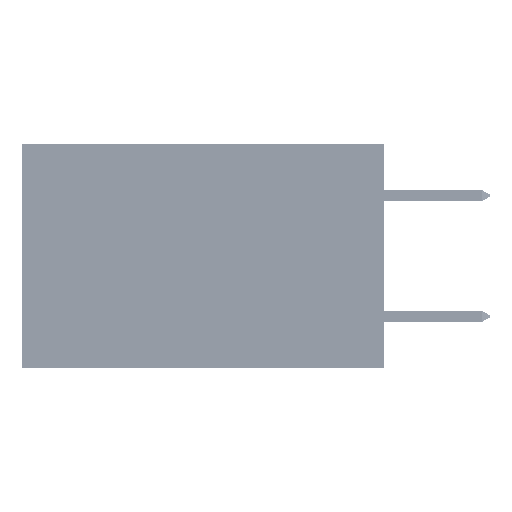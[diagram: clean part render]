
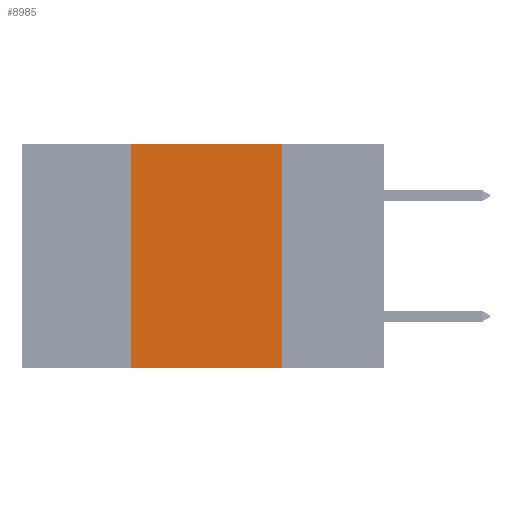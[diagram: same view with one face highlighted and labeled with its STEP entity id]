
A CAD part, left-side view. The second image highlights one B-rep face of the part: STEP entity #8985.
In plain terms, the highlighted planar face has unit normal (-1, 0, 0).
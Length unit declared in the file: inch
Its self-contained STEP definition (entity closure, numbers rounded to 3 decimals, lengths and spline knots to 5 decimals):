
#1843 = ORIENTED_EDGE ( 'NONE', *, *, #11566, .F. ) ;
#3091 = CARTESIAN_POINT ( 'NONE',  ( 0., 0.6, 0. ) ) ;
#4991 = CARTESIAN_POINT ( 'NONE',  ( 0., 0.17, 0. ) ) ;
#5970 = DIRECTION ( 'NONE',  ( 0., -1., 0. ) ) ;
#8985 = ADVANCED_FACE ( 'NONE', ( #24442 ), #37626, .F. ) ;
#10813 = DIRECTION ( 'NONE',  ( 0., 0., -1. ) ) ;
#11566 = EDGE_CURVE ( 'NONE', #29996, #33161, #38709, .T. ) ;
#12759 = LINE ( 'NONE', #25052, #21851 ) ;
#14288 = VERTEX_POINT ( 'NONE', #33028 ) ;
#17125 = LINE ( 'NONE', #33370, #24985 ) ;
#18031 = AXIS2_PLACEMENT_3D ( 'NONE', #3091, #33879, #10813 ) ;
#18516 = CARTESIAN_POINT ( 'NONE',  ( 0., 0.17, -0.37 ) ) ;
#21851 = VECTOR ( 'NONE', #5970, 39.37008 ) ;
#21865 = DIRECTION ( 'NONE',  ( 0., 0., 1. ) ) ;
#23461 = EDGE_CURVE ( 'NONE', #41573, #29996, #12759, .T. ) ;
#24442 = FACE_OUTER_BOUND ( 'NONE', #39516, .T. ) ;
#24985 = VECTOR ( 'NONE', #45136, 39.37008 ) ;
#25052 = CARTESIAN_POINT ( 'NONE',  ( 0., 0.6, 0. ) ) ;
#26537 = VECTOR ( 'NONE', #21865, 39.37008 ) ;
#29996 = VERTEX_POINT ( 'NONE', #35547 ) ;
#30983 = ORIENTED_EDGE ( 'NONE', *, *, #23461, .F. ) ;
#33028 = CARTESIAN_POINT ( 'NONE',  ( 0., 0.42, -0.37 ) ) ;
#33161 = VERTEX_POINT ( 'NONE', #18516 ) ;
#33370 = CARTESIAN_POINT ( 'NONE',  ( 0., 0.6, -0.37 ) ) ;
#33635 = CARTESIAN_POINT ( 'NONE',  ( 0., 0.42, 0. ) ) ;
#33879 = DIRECTION ( 'NONE',  ( 1., 0., 0. ) ) ;
#34539 = ORIENTED_EDGE ( 'NONE', *, *, #34714, .F. ) ;
#34714 = EDGE_CURVE ( 'NONE', #14288, #41573, #37974, .T. ) ;
#35547 = CARTESIAN_POINT ( 'NONE',  ( 0., 0.17, 0. ) ) ;
#37479 = VECTOR ( 'NONE', #47565, 39.37008 ) ;
#37626 = PLANE ( 'NONE',  #18031 ) ;
#37974 = LINE ( 'NONE', #41105, #26537 ) ;
#38709 = LINE ( 'NONE', #4991, #37479 ) ;
#39516 = EDGE_LOOP ( 'NONE', ( #1843, #30983, #34539, #43052 ) ) ;
#41105 = CARTESIAN_POINT ( 'NONE',  ( 0., 0.42, 0. ) ) ;
#41573 = VERTEX_POINT ( 'NONE', #33635 ) ;
#43052 = ORIENTED_EDGE ( 'NONE', *, *, #45063, .T. ) ;
#45063 = EDGE_CURVE ( 'NONE', #14288, #33161, #17125, .T. ) ;
#45136 = DIRECTION ( 'NONE',  ( 0., -1., 0. ) ) ;
#47565 = DIRECTION ( 'NONE',  ( 0., 0., -1. ) ) ;
